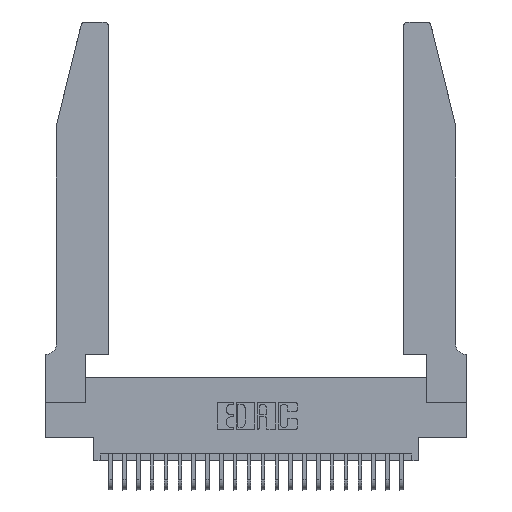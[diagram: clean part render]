
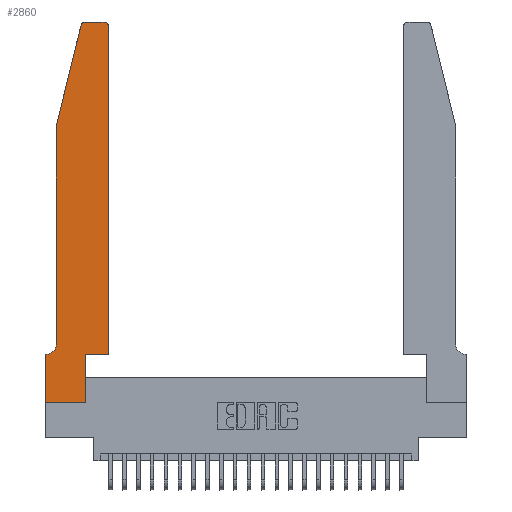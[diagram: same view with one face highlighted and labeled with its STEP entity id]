
A CAD part, top view. The second image highlights one B-rep face of the part: STEP entity #2860.
In plain terms, the highlighted planar face has unit normal (0, 0, 1).
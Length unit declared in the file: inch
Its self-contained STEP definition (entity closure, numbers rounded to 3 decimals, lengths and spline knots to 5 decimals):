
#544 = EDGE_CURVE ( 'NONE', #16553, #2627, #21071, .T. ) ;
#810 = DIRECTION ( 'NONE',  ( 0., 1., 0. ) ) ;
#1020 = VERTEX_POINT ( 'NONE', #17325 ) ;
#1097 = DIRECTION ( 'NONE',  ( -1., 0., 0. ) ) ;
#1173 = ORIENTED_EDGE ( 'NONE', *, *, #13770, .T. ) ;
#1474 = CARTESIAN_POINT ( 'NONE',  ( 0., 0.35, 0.37 ) ) ;
#1793 = CARTESIAN_POINT ( 'NONE',  ( 0.2865, 0.35, 0.37 ) ) ;
#2051 = CARTESIAN_POINT ( 'NONE',  ( 0.0755, 0.42, 0.37 ) ) ;
#2281 = DIRECTION ( 'NONE',  ( 1., 0., 0. ) ) ;
#2286 = ORIENTED_EDGE ( 'NONE', *, *, #21392, .T. ) ;
#2326 = VECTOR ( 'NONE', #22865, 39.37008 ) ;
#2549 = EDGE_CURVE ( 'NONE', #22711, #6148, #19071, .T. ) ;
#2606 = CARTESIAN_POINT ( 'NONE',  ( 0., 0., 0.37 ) ) ;
#2627 = VERTEX_POINT ( 'NONE', #10942 ) ;
#2630 = AXIS2_PLACEMENT_3D ( 'NONE', #25201, #19233, #12894 ) ;
#2668 = CARTESIAN_POINT ( 'NONE',  ( 0.2865, 0.35, 0.37 ) ) ;
#2860 = ADVANCED_FACE ( 'NONE', ( #23541 ), #3531, .T. ) ;
#3034 = ORIENTED_EDGE ( 'NONE', *, *, #12256, .T. ) ;
#3101 = EDGE_CURVE ( 'NONE', #8924, #23765, #23521, .T. ) ;
#3295 = DIRECTION ( 'NONE',  ( 0., -1., 0. ) ) ;
#3531 = PLANE ( 'NONE',  #23057 ) ;
#3610 = CARTESIAN_POINT ( 'NONE',  ( 0.4505, 0.35, 0.37 ) ) ;
#3637 = DIRECTION ( 'NONE',  ( 0., 0., -1. ) ) ;
#3691 = DIRECTION ( 'NONE',  ( 1., 0., 0. ) ) ;
#3883 = DIRECTION ( 'NONE',  ( -1., 0., 0. ) ) ;
#4098 = LINE ( 'NONE', #3610, #14951 ) ;
#4522 = DIRECTION ( 'NONE',  ( 0., 0., 1. ) ) ;
#4703 = LINE ( 'NONE', #21418, #5991 ) ;
#5602 = DIRECTION ( 'NONE',  ( -1., 0., 0. ) ) ;
#5926 = CARTESIAN_POINT ( 'NONE',  ( 0.0755, 2., 0.37 ) ) ;
#5946 = LINE ( 'NONE', #2668, #11371 ) ;
#5991 = VECTOR ( 'NONE', #3295, 39.37008 ) ;
#6148 = VERTEX_POINT ( 'NONE', #11997 ) ;
#6484 = EDGE_CURVE ( 'NONE', #6148, #8770, #18704, .T. ) ;
#6693 = LINE ( 'NONE', #17140, #7650 ) ;
#7303 = VERTEX_POINT ( 'NONE', #10389 ) ;
#7448 = LINE ( 'NONE', #18857, #2326 ) ;
#7650 = VECTOR ( 'NONE', #1097, 39.37008 ) ;
#8430 = VECTOR ( 'NONE', #24046, 39.37008 ) ;
#8770 = VERTEX_POINT ( 'NONE', #21504 ) ;
#8924 = VERTEX_POINT ( 'NONE', #2606 ) ;
#9007 = ORIENTED_EDGE ( 'NONE', *, *, #25377, .T. ) ;
#9279 = ORIENTED_EDGE ( 'NONE', *, *, #3101, .T. ) ;
#9632 = CARTESIAN_POINT ( 'NONE',  ( 0.0055, 0.42, 0.37 ) ) ;
#9804 = LINE ( 'NONE', #11616, #25881 ) ;
#9839 = EDGE_CURVE ( 'NONE', #16551, #7303, #6693, .T. ) ;
#10333 = DIRECTION ( 'NONE',  ( 1., 0., 0. ) ) ;
#10389 = CARTESIAN_POINT ( 'NONE',  ( 0., 0.35, 0.37 ) ) ;
#10881 = CARTESIAN_POINT ( 'NONE',  ( 0.284, 2.75, 0.37 ) ) ;
#10936 = VERTEX_POINT ( 'NONE', #1793 ) ;
#10942 = CARTESIAN_POINT ( 'NONE',  ( 0.4205, 2.75, 0.37 ) ) ;
#11371 = VECTOR ( 'NONE', #810, 39.37008 ) ;
#11576 = DIRECTION ( 'NONE',  ( 0., 0., 1. ) ) ;
#11616 = CARTESIAN_POINT ( 'NONE',  ( 0., 0., 0.37 ) ) ;
#11997 = CARTESIAN_POINT ( 'NONE',  ( 0.25487, 2.72718, 0.37 ) ) ;
#12256 = EDGE_CURVE ( 'NONE', #8770, #22350, #4703, .T. ) ;
#12415 = AXIS2_PLACEMENT_3D ( 'NONE', #16797, #4522, #2281 ) ;
#12894 = DIRECTION ( 'NONE',  ( 1., 0., 0. ) ) ;
#13400 = ORIENTED_EDGE ( 'NONE', *, *, #20732, .T. ) ;
#13770 = EDGE_CURVE ( 'NONE', #23765, #10936, #5946, .T. ) ;
#14022 = EDGE_LOOP ( 'NONE', ( #13400, #25276, #18612, #3034, #21057, #18596, #9007, #9279, #1173, #18174, #2286, #20419 ) ) ;
#14951 = VECTOR ( 'NONE', #3691, 39.37008 ) ;
#15511 = DIRECTION ( 'NONE',  ( 1., 0., 0. ) ) ;
#16386 = CARTESIAN_POINT ( 'NONE',  ( 0.4505, 2.72, 0.37 ) ) ;
#16551 = VERTEX_POINT ( 'NONE', #25466 ) ;
#16553 = VERTEX_POINT ( 'NONE', #16386 ) ;
#16797 = CARTESIAN_POINT ( 'NONE',  ( 0.284, 2.72, 0.37 ) ) ;
#17140 = CARTESIAN_POINT ( 'NONE',  ( 0.0755, 0.35, 0.37 ) ) ;
#17325 = CARTESIAN_POINT ( 'NONE',  ( 0.4505, 0.35, 0.37 ) ) ;
#18174 = ORIENTED_EDGE ( 'NONE', *, *, #24846, .T. ) ;
#18596 = ORIENTED_EDGE ( 'NONE', *, *, #9839, .T. ) ;
#18612 = ORIENTED_EDGE ( 'NONE', *, *, #6484, .T. ) ;
#18704 = LINE ( 'NONE', #5926, #8430 ) ;
#18857 = CARTESIAN_POINT ( 'NONE',  ( 0.4505, 0.35, 0.37 ) ) ;
#19058 = VECTOR ( 'NONE', #3883, 39.37008 ) ;
#19071 = CIRCLE ( 'NONE', #12415, 0.03 ) ;
#19083 = CIRCLE ( 'NONE', #25758, 0.07 ) ;
#19233 = DIRECTION ( 'NONE',  ( 0., 0., 1. ) ) ;
#19537 = DIRECTION ( 'NONE',  ( 0., -1., 0. ) ) ;
#19715 = LINE ( 'NONE', #22331, #19058 ) ;
#20000 = EDGE_CURVE ( 'NONE', #22350, #16551, #19083, .T. ) ;
#20419 = ORIENTED_EDGE ( 'NONE', *, *, #544, .T. ) ;
#20500 = CARTESIAN_POINT ( 'NONE',  ( 0., 0., 0.37 ) ) ;
#20732 = EDGE_CURVE ( 'NONE', #2627, #22711, #19715, .T. ) ;
#21057 = ORIENTED_EDGE ( 'NONE', *, *, #20000, .T. ) ;
#21071 = CIRCLE ( 'NONE', #2630, 0.03 ) ;
#21392 = EDGE_CURVE ( 'NONE', #1020, #16553, #7448, .T. ) ;
#21418 = CARTESIAN_POINT ( 'NONE',  ( 0.0755, 2., 0.37 ) ) ;
#21504 = CARTESIAN_POINT ( 'NONE',  ( 0.0755, 2., 0.37 ) ) ;
#22331 = CARTESIAN_POINT ( 'NONE',  ( 0.2605, 2.75, 0.37 ) ) ;
#22350 = VERTEX_POINT ( 'NONE', #2051 ) ;
#22711 = VERTEX_POINT ( 'NONE', #10881 ) ;
#22738 = CARTESIAN_POINT ( 'NONE',  ( 0.2865, 0., 0.37 ) ) ;
#22865 = DIRECTION ( 'NONE',  ( 0., 1., 0. ) ) ;
#23057 = AXIS2_PLACEMENT_3D ( 'NONE', #1474, #11576, #15511 ) ;
#23521 = LINE ( 'NONE', #20500, #26122 ) ;
#23541 = FACE_OUTER_BOUND ( 'NONE', #14022, .T. ) ;
#23765 = VERTEX_POINT ( 'NONE', #22738 ) ;
#24046 = DIRECTION ( 'NONE',  ( -0.239, -0.971, 0. ) ) ;
#24846 = EDGE_CURVE ( 'NONE', #10936, #1020, #4098, .T. ) ;
#25201 = CARTESIAN_POINT ( 'NONE',  ( 0.4205, 2.72, 0.37 ) ) ;
#25276 = ORIENTED_EDGE ( 'NONE', *, *, #2549, .T. ) ;
#25377 = EDGE_CURVE ( 'NONE', #7303, #8924, #9804, .T. ) ;
#25466 = CARTESIAN_POINT ( 'NONE',  ( 0.0055, 0.35, 0.37 ) ) ;
#25758 = AXIS2_PLACEMENT_3D ( 'NONE', #9632, #3637, #5602 ) ;
#25881 = VECTOR ( 'NONE', #19537, 39.37008 ) ;
#26122 = VECTOR ( 'NONE', #10333, 39.37008 ) ;
